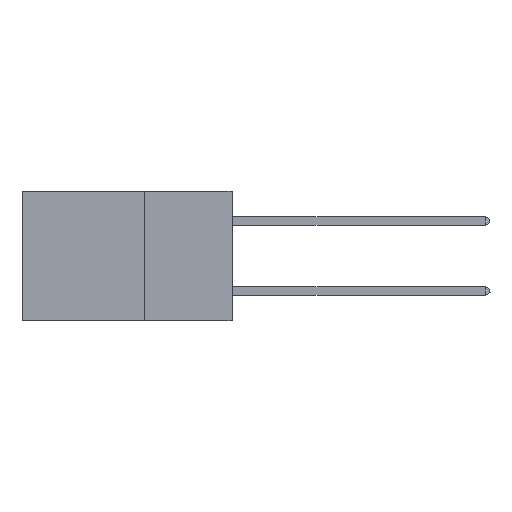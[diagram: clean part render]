
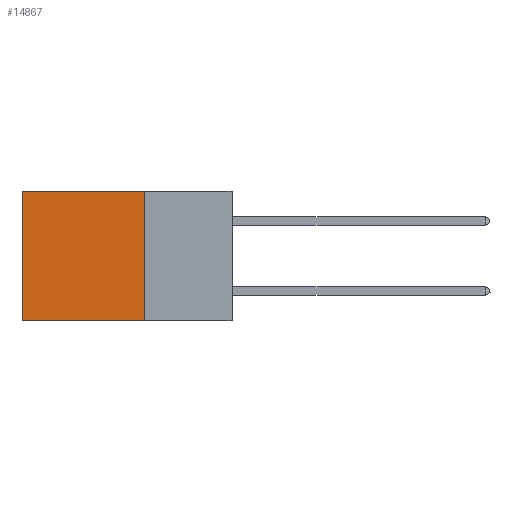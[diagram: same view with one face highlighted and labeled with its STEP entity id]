
A CAD part, left-side view. The second image highlights one B-rep face of the part: STEP entity #14867.
In plain terms, the highlighted planar face has unit normal (-1, 0, 0).
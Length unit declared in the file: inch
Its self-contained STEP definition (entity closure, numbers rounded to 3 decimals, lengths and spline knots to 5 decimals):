
#213 = CARTESIAN_POINT ( 'NONE',  ( 0.2875, 0.25, -0.37 ) ) ;
#446 = LINE ( 'NONE', #10697, #21736 ) ;
#2374 = CARTESIAN_POINT ( 'NONE',  ( 0.2875, 0.25, 0. ) ) ;
#3173 = EDGE_CURVE ( 'NONE', #19381, #14529, #7636, .T. ) ;
#3249 = VERTEX_POINT ( 'NONE', #19331 ) ;
#3968 = CARTESIAN_POINT ( 'NONE',  ( 0.2875, 0.25, 0. ) ) ;
#4817 = EDGE_CURVE ( 'NONE', #19381, #3249, #446, .T. ) ;
#6855 = CARTESIAN_POINT ( 'NONE',  ( 0.2875, 0.6, 0. ) ) ;
#7636 = LINE ( 'NONE', #3968, #16095 ) ;
#7983 = CARTESIAN_POINT ( 'NONE',  ( 0.2875, 0.25, -0.37 ) ) ;
#8437 = ORIENTED_EDGE ( 'NONE', *, *, #4817, .T. ) ;
#8844 = DIRECTION ( 'NONE',  ( 0., 1., 0. ) ) ;
#9952 = ORIENTED_EDGE ( 'NONE', *, *, #16678, .T. ) ;
#10026 = CARTESIAN_POINT ( 'NONE',  ( 0.2875, 0.25, 0. ) ) ;
#10697 = CARTESIAN_POINT ( 'NONE',  ( 0.2875, 0.25, 0. ) ) ;
#12015 = ORIENTED_EDGE ( 'NONE', *, *, #13406, .F. ) ;
#12204 = VECTOR ( 'NONE', #8844, 39.37008 ) ;
#12436 = DIRECTION ( 'NONE',  ( 0., 1., 0. ) ) ;
#13406 = EDGE_CURVE ( 'NONE', #14529, #17669, #17412, .T. ) ;
#13849 = AXIS2_PLACEMENT_3D ( 'NONE', #2374, #19713, #19941 ) ;
#14314 = CARTESIAN_POINT ( 'NONE',  ( 0.2875, 0.6, -0.37 ) ) ;
#14529 = VERTEX_POINT ( 'NONE', #7983 ) ;
#14867 = ADVANCED_FACE ( 'NONE', ( #20062 ), #16442, .F. ) ;
#16095 = VECTOR ( 'NONE', #19648, 39.37008 ) ;
#16429 = LINE ( 'NONE', #6855, #16714 ) ;
#16442 = PLANE ( 'NONE',  #13849 ) ;
#16678 = EDGE_CURVE ( 'NONE', #3249, #17669, #16429, .T. ) ;
#16714 = VECTOR ( 'NONE', #20637, 39.37008 ) ;
#17038 = ORIENTED_EDGE ( 'NONE', *, *, #3173, .F. ) ;
#17412 = LINE ( 'NONE', #213, #12204 ) ;
#17669 = VERTEX_POINT ( 'NONE', #14314 ) ;
#18757 = EDGE_LOOP ( 'NONE', ( #9952, #12015, #17038, #8437 ) ) ;
#19331 = CARTESIAN_POINT ( 'NONE',  ( 0.2875, 0.6, 0. ) ) ;
#19381 = VERTEX_POINT ( 'NONE', #10026 ) ;
#19648 = DIRECTION ( 'NONE',  ( 0., 0., -1. ) ) ;
#19713 = DIRECTION ( 'NONE',  ( 1., 0., 0. ) ) ;
#19941 = DIRECTION ( 'NONE',  ( 0., 0., -1. ) ) ;
#20062 = FACE_OUTER_BOUND ( 'NONE', #18757, .T. ) ;
#20637 = DIRECTION ( 'NONE',  ( 0., 0., -1. ) ) ;
#21736 = VECTOR ( 'NONE', #12436, 39.37008 ) ;
